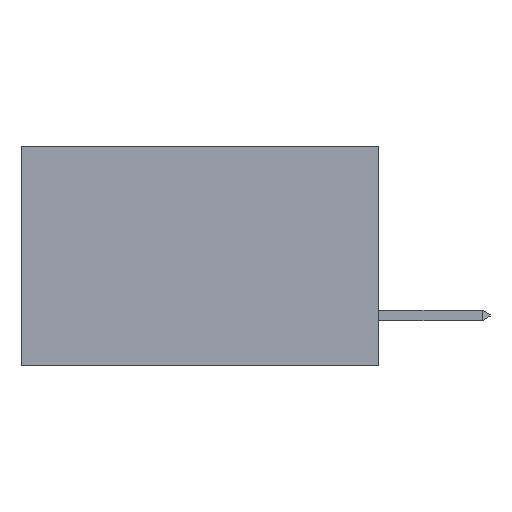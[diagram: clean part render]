
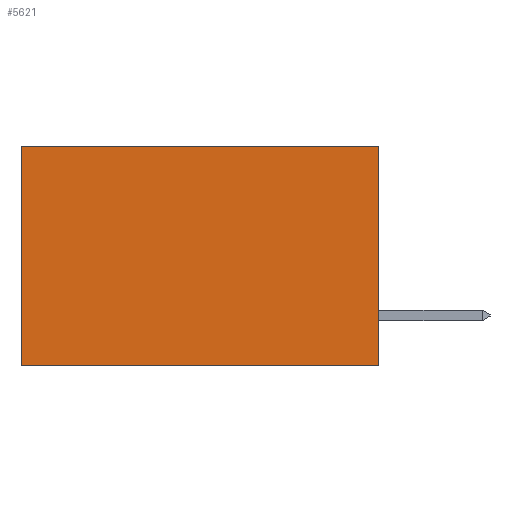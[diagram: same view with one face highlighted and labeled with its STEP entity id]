
A CAD part, left-side view. The second image highlights one B-rep face of the part: STEP entity #5621.
In plain terms, the highlighted planar face has unit normal (-1, 0, 0).
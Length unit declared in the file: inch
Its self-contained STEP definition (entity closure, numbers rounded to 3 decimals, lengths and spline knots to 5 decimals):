
#294 = DIRECTION ( 'NONE',  ( 0., 1., 0. ) ) ;
#484 = CARTESIAN_POINT ( 'NONE',  ( 0.2615, 0., -0.37 ) ) ;
#1370 = ORIENTED_EDGE ( 'NONE', *, *, #10548, .T. ) ;
#1483 = VERTEX_POINT ( 'NONE', #5443 ) ;
#1585 = CARTESIAN_POINT ( 'NONE',  ( 0.2615, 0., -0.37 ) ) ;
#3889 = ORIENTED_EDGE ( 'NONE', *, *, #8758, .F. ) ;
#4043 = VERTEX_POINT ( 'NONE', #15068 ) ;
#4403 = VECTOR ( 'NONE', #294, 39.37008 ) ;
#5140 = EDGE_CURVE ( 'NONE', #6973, #4043, #14605, .T. ) ;
#5217 = FACE_OUTER_BOUND ( 'NONE', #5591, .T. ) ;
#5382 = DIRECTION ( 'NONE',  ( 0., 1., 0. ) ) ;
#5443 = CARTESIAN_POINT ( 'NONE',  ( 0.2615, 0., 0. ) ) ;
#5591 = EDGE_LOOP ( 'NONE', ( #15712, #7068, #3889, #1370 ) ) ;
#5621 = ADVANCED_FACE ( 'NONE', ( #5217 ), #14835, .F. ) ;
#6866 = DIRECTION ( 'NONE',  ( 0., 0., -1. ) ) ;
#6973 = VERTEX_POINT ( 'NONE', #10861 ) ;
#7068 = ORIENTED_EDGE ( 'NONE', *, *, #13633, .F. ) ;
#7335 = CARTESIAN_POINT ( 'NONE',  ( 0.2615, 0.6, -0.37 ) ) ;
#8011 = VERTEX_POINT ( 'NONE', #484 ) ;
#8165 = VECTOR ( 'NONE', #9419, 39.37008 ) ;
#8606 = VECTOR ( 'NONE', #5382, 39.37008 ) ;
#8758 = EDGE_CURVE ( 'NONE', #1483, #8011, #9135, .T. ) ;
#9135 = LINE ( 'NONE', #9311, #15877 ) ;
#9311 = CARTESIAN_POINT ( 'NONE',  ( 0.2615, 0., -0.37 ) ) ;
#9419 = DIRECTION ( 'NONE',  ( 0., 0., -1. ) ) ;
#10548 = EDGE_CURVE ( 'NONE', #1483, #6973, #14567, .T. ) ;
#10861 = CARTESIAN_POINT ( 'NONE',  ( 0.2615, 0.6, 0. ) ) ;
#11479 = LINE ( 'NONE', #1585, #8606 ) ;
#11495 = CARTESIAN_POINT ( 'NONE',  ( 0.2615, 0., 0. ) ) ;
#13096 = AXIS2_PLACEMENT_3D ( 'NONE', #14724, #14711, #14656 ) ;
#13633 = EDGE_CURVE ( 'NONE', #8011, #4043, #11479, .T. ) ;
#14567 = LINE ( 'NONE', #11495, #4403 ) ;
#14605 = LINE ( 'NONE', #7335, #8165 ) ;
#14656 = DIRECTION ( 'NONE',  ( 0., 0., -1. ) ) ;
#14711 = DIRECTION ( 'NONE',  ( 1., 0., 0. ) ) ;
#14724 = CARTESIAN_POINT ( 'NONE',  ( 0.2615, 0., -0.37 ) ) ;
#14835 = PLANE ( 'NONE',  #13096 ) ;
#15068 = CARTESIAN_POINT ( 'NONE',  ( 0.2615, 0.6, -0.37 ) ) ;
#15712 = ORIENTED_EDGE ( 'NONE', *, *, #5140, .T. ) ;
#15877 = VECTOR ( 'NONE', #6866, 39.37008 ) ;
